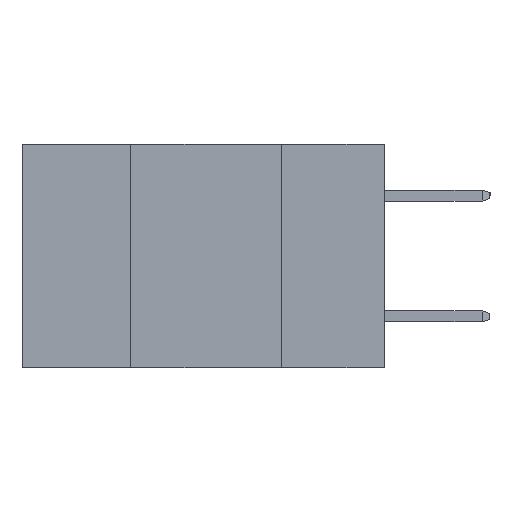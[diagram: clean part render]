
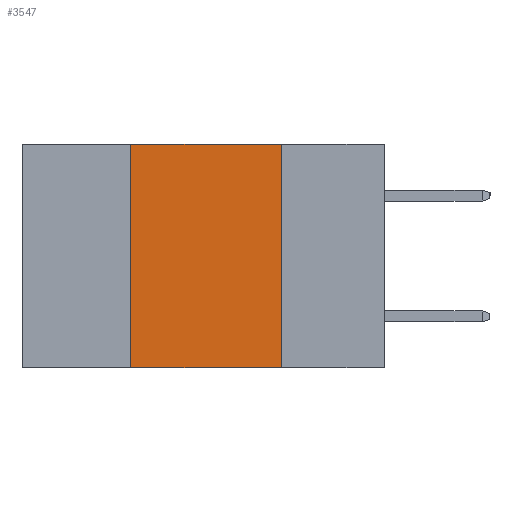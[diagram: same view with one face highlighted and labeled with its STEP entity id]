
A CAD part, left-side view. The second image highlights one B-rep face of the part: STEP entity #3547.
In plain terms, the highlighted planar face has unit normal (-1, 0, 0).
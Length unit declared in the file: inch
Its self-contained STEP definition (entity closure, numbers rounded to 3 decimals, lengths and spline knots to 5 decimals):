
#1085 = DIRECTION ( 'NONE',  ( 1., 0., 0. ) ) ;
#1237 = DIRECTION ( 'NONE',  ( 0., 0., -1. ) ) ;
#1893 = VERTEX_POINT ( 'NONE', #5300 ) ;
#2017 = CARTESIAN_POINT ( 'NONE',  ( 0., 0.42, 0. ) ) ;
#2474 = VECTOR ( 'NONE', #3584, 39.37008 ) ;
#2876 = LINE ( 'NONE', #4987, #10039 ) ;
#3429 = EDGE_CURVE ( 'NONE', #8314, #11077, #5538, .T. ) ;
#3547 = ADVANCED_FACE ( 'NONE', ( #4489 ), #6813, .F. ) ;
#3584 = DIRECTION ( 'NONE',  ( 0., -1., 0. ) ) ;
#3970 = ORIENTED_EDGE ( 'NONE', *, *, #5532, .T. ) ;
#4489 = FACE_OUTER_BOUND ( 'NONE', #9300, .T. ) ;
#4987 = CARTESIAN_POINT ( 'NONE',  ( 0., 0.6, -0.37 ) ) ;
#5151 = LINE ( 'NONE', #12186, #9161 ) ;
#5300 = CARTESIAN_POINT ( 'NONE',  ( 0., 0.17, -0.37 ) ) ;
#5485 = CARTESIAN_POINT ( 'NONE',  ( 0., 0.42, -0.37 ) ) ;
#5532 = EDGE_CURVE ( 'NONE', #8314, #1893, #2876, .T. ) ;
#5538 = LINE ( 'NONE', #13639, #6162 ) ;
#6162 = VECTOR ( 'NONE', #10229, 39.37008 ) ;
#6813 = PLANE ( 'NONE',  #7368 ) ;
#6995 = CARTESIAN_POINT ( 'NONE',  ( 0., 0.17, 0. ) ) ;
#7368 = AXIS2_PLACEMENT_3D ( 'NONE', #11647, #1085, #1237 ) ;
#7394 = DIRECTION ( 'NONE',  ( 0., -1., 0. ) ) ;
#8314 = VERTEX_POINT ( 'NONE', #5485 ) ;
#9115 = CARTESIAN_POINT ( 'NONE',  ( 0., 0.6, 0. ) ) ;
#9161 = VECTOR ( 'NONE', #9780, 39.37008 ) ;
#9300 = EDGE_LOOP ( 'NONE', ( #11178, #13467, #9957, #3970 ) ) ;
#9780 = DIRECTION ( 'NONE',  ( 0., 0., -1. ) ) ;
#9957 = ORIENTED_EDGE ( 'NONE', *, *, #3429, .F. ) ;
#10039 = VECTOR ( 'NONE', #7394, 39.37008 ) ;
#10229 = DIRECTION ( 'NONE',  ( 0., 0., 1. ) ) ;
#10755 = VERTEX_POINT ( 'NONE', #6995 ) ;
#11077 = VERTEX_POINT ( 'NONE', #2017 ) ;
#11178 = ORIENTED_EDGE ( 'NONE', *, *, #11523, .F. ) ;
#11523 = EDGE_CURVE ( 'NONE', #10755, #1893, #5151, .T. ) ;
#11647 = CARTESIAN_POINT ( 'NONE',  ( 0., 0.6, 0. ) ) ;
#11661 = LINE ( 'NONE', #9115, #2474 ) ;
#12186 = CARTESIAN_POINT ( 'NONE',  ( 0., 0.17, -0.37 ) ) ;
#13467 = ORIENTED_EDGE ( 'NONE', *, *, #14889, .F. ) ;
#13639 = CARTESIAN_POINT ( 'NONE',  ( 0., 0.42, -0.37 ) ) ;
#14889 = EDGE_CURVE ( 'NONE', #11077, #10755, #11661, .T. ) ;
